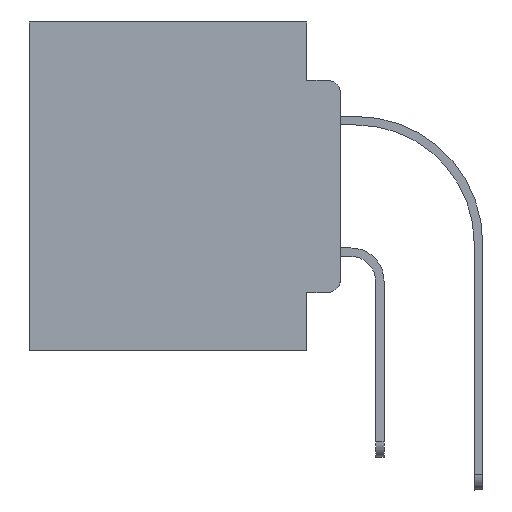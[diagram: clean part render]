
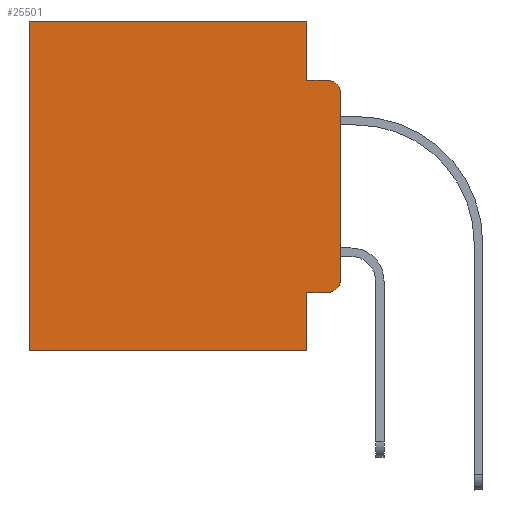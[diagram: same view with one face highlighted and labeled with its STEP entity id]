
A CAD part, left-side view. The second image highlights one B-rep face of the part: STEP entity #25501.
In plain terms, the highlighted planar face has unit normal (-1, 0, 0).
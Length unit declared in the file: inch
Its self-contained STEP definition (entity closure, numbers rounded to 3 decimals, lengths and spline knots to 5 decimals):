
#124 = DIRECTION ( 'NONE',  ( 1., 0., 0. ) ) ;
#854 = CARTESIAN_POINT ( 'NONE',  ( 0.298, 0.051, -0.5 ) ) ;
#1915 = VERTEX_POINT ( 'NONE', #29930 ) ;
#1949 = CARTESIAN_POINT ( 'NONE',  ( 0.298, 0., 0. ) ) ;
#2885 = DIRECTION ( 'NONE',  ( 0., 0., -1. ) ) ;
#4285 = DIRECTION ( 'NONE',  ( 0., 0., -1. ) ) ;
#4287 = EDGE_CURVE ( 'NONE', #28174, #19011, #19412, .T. ) ;
#4570 = CARTESIAN_POINT ( 'NONE',  ( 0.298, 0.02, -0.3915 ) ) ;
#4845 = DIRECTION ( 'NONE',  ( 0., 1., 0. ) ) ;
#4975 = LINE ( 'NONE', #23577, #9505 ) ;
#5731 = LINE ( 'NONE', #26779, #25128 ) ;
#6683 = VERTEX_POINT ( 'NONE', #12131 ) ;
#6685 = ORIENTED_EDGE ( 'NONE', *, *, #4287, .T. ) ;
#6766 = AXIS2_PLACEMENT_3D ( 'NONE', #4570, #13886, #18301 ) ;
#7249 = DIRECTION ( 'NONE',  ( 0., 0., -1. ) ) ;
#8041 = AXIS2_PLACEMENT_3D ( 'NONE', #26088, #9938, #25486 ) ;
#8738 = CARTESIAN_POINT ( 'NONE',  ( 0.298, 0., -0.1085 ) ) ;
#8766 = VERTEX_POINT ( 'NONE', #854 ) ;
#9167 = VERTEX_POINT ( 'NONE', #28833 ) ;
#9399 = CARTESIAN_POINT ( 'NONE',  ( 0.298, 0.051, 0. ) ) ;
#9505 = VECTOR ( 'NONE', #21282, 39.37008 ) ;
#9827 = AXIS2_PLACEMENT_3D ( 'NONE', #1949, #124, #11269 ) ;
#9938 = DIRECTION ( 'NONE',  ( -1., 0., 0. ) ) ;
#10258 = EDGE_CURVE ( 'NONE', #20858, #19011, #5731, .T. ) ;
#10445 = CIRCLE ( 'NONE', #8041, 0.02 ) ;
#11269 = DIRECTION ( 'NONE',  ( 0., 0., -1. ) ) ;
#11733 = ORIENTED_EDGE ( 'NONE', *, *, #20547, .F. ) ;
#11778 = LINE ( 'NONE', #22741, #14499 ) ;
#11998 = ORIENTED_EDGE ( 'NONE', *, *, #15380, .T. ) ;
#12131 = CARTESIAN_POINT ( 'NONE',  ( 0.298, 0.473, -0.5 ) ) ;
#12573 = LINE ( 'NONE', #18399, #17850 ) ;
#12671 = CARTESIAN_POINT ( 'NONE',  ( 0.298, 0.02, -0.0885 ) ) ;
#12758 = ORIENTED_EDGE ( 'NONE', *, *, #18833, .F. ) ;
#13554 = PLANE ( 'NONE',  #9827 ) ;
#13886 = DIRECTION ( 'NONE',  ( -1., 0., 0. ) ) ;
#14499 = VECTOR ( 'NONE', #4285, 39.37008 ) ;
#14501 = ORIENTED_EDGE ( 'NONE', *, *, #16462, .F. ) ;
#15380 = EDGE_CURVE ( 'NONE', #9167, #28174, #23101, .T. ) ;
#15548 = EDGE_LOOP ( 'NONE', ( #17728, #18456, #12758, #26616, #26475, #19724, #11733, #14501, #11998, #6685 ) ) ;
#15975 = VECTOR ( 'NONE', #2885, 39.37008 ) ;
#16274 = DIRECTION ( 'NONE',  ( 0., 1., 0. ) ) ;
#16462 = EDGE_CURVE ( 'NONE', #9167, #8766, #19209, .T. ) ;
#17235 = CARTESIAN_POINT ( 'NONE',  ( 0.298, 0.051, 0. ) ) ;
#17728 = ORIENTED_EDGE ( 'NONE', *, *, #10258, .F. ) ;
#17850 = VECTOR ( 'NONE', #16274, 39.37008 ) ;
#18128 = FACE_OUTER_BOUND ( 'NONE', #15548, .T. ) ;
#18271 = CARTESIAN_POINT ( 'NONE',  ( 0.298, 0., 0. ) ) ;
#18301 = DIRECTION ( 'NONE',  ( 0., 0., -1. ) ) ;
#18330 = EDGE_CURVE ( 'NONE', #20858, #26459, #10445, .T. ) ;
#18399 = CARTESIAN_POINT ( 'NONE',  ( 0.298, 0., -0.5 ) ) ;
#18413 = LINE ( 'NONE', #18271, #28817 ) ;
#18456 = ORIENTED_EDGE ( 'NONE', *, *, #18330, .T. ) ;
#18826 = LINE ( 'NONE', #9399, #26132 ) ;
#18833 = EDGE_CURVE ( 'NONE', #1915, #26459, #4975, .T. ) ;
#19011 = VERTEX_POINT ( 'NONE', #29043 ) ;
#19209 = LINE ( 'NONE', #28653, #15975 ) ;
#19412 = CIRCLE ( 'NONE', #6766, 0.02 ) ;
#19617 = VECTOR ( 'NONE', #25399, 39.37008 ) ;
#19724 = ORIENTED_EDGE ( 'NONE', *, *, #29377, .T. ) ;
#20547 = EDGE_CURVE ( 'NONE', #8766, #6683, #12573, .T. ) ;
#20649 = CARTESIAN_POINT ( 'NONE',  ( 0.298, 0.473, 0. ) ) ;
#20858 = VERTEX_POINT ( 'NONE', #8738 ) ;
#21265 = CARTESIAN_POINT ( 'NONE',  ( 0.298, 0.051, -0.4115 ) ) ;
#21282 = DIRECTION ( 'NONE',  ( 0., -1., 0. ) ) ;
#22251 = EDGE_CURVE ( 'NONE', #22869, #1915, #18826, .T. ) ;
#22741 = CARTESIAN_POINT ( 'NONE',  ( 0.298, 0.473, 0. ) ) ;
#22869 = VERTEX_POINT ( 'NONE', #17235 ) ;
#23101 = LINE ( 'NONE', #21265, #19617 ) ;
#23577 = CARTESIAN_POINT ( 'NONE',  ( 0.298, 0.051, -0.0885 ) ) ;
#24340 = DIRECTION ( 'NONE',  ( 0., 0., -1. ) ) ;
#25128 = VECTOR ( 'NONE', #24340, 39.37008 ) ;
#25241 = VERTEX_POINT ( 'NONE', #20649 ) ;
#25372 = EDGE_CURVE ( 'NONE', #22869, #25241, #18413, .T. ) ;
#25399 = DIRECTION ( 'NONE',  ( 0., -1., 0. ) ) ;
#25486 = DIRECTION ( 'NONE',  ( 0., 0., -1. ) ) ;
#25501 = ADVANCED_FACE ( 'NONE', ( #18128 ), #13554, .F. ) ;
#26088 = CARTESIAN_POINT ( 'NONE',  ( 0.298, 0.02, -0.1085 ) ) ;
#26132 = VECTOR ( 'NONE', #7249, 39.37008 ) ;
#26239 = CARTESIAN_POINT ( 'NONE',  ( 0.298, 0.02, -0.4115 ) ) ;
#26459 = VERTEX_POINT ( 'NONE', #12671 ) ;
#26475 = ORIENTED_EDGE ( 'NONE', *, *, #25372, .T. ) ;
#26616 = ORIENTED_EDGE ( 'NONE', *, *, #22251, .F. ) ;
#26779 = CARTESIAN_POINT ( 'NONE',  ( 0.298, 0., 0. ) ) ;
#28174 = VERTEX_POINT ( 'NONE', #26239 ) ;
#28653 = CARTESIAN_POINT ( 'NONE',  ( 0.298, 0.051, 0. ) ) ;
#28817 = VECTOR ( 'NONE', #4845, 39.37008 ) ;
#28833 = CARTESIAN_POINT ( 'NONE',  ( 0.298, 0.051, -0.4115 ) ) ;
#29043 = CARTESIAN_POINT ( 'NONE',  ( 0.298, 0., -0.3915 ) ) ;
#29377 = EDGE_CURVE ( 'NONE', #25241, #6683, #11778, .T. ) ;
#29930 = CARTESIAN_POINT ( 'NONE',  ( 0.298, 0.051, -0.0885 ) ) ;
